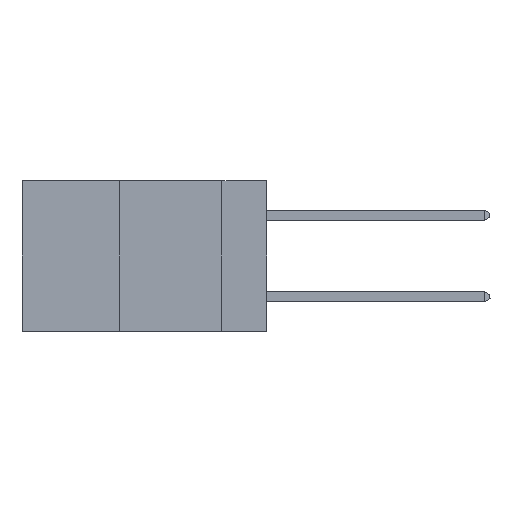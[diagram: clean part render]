
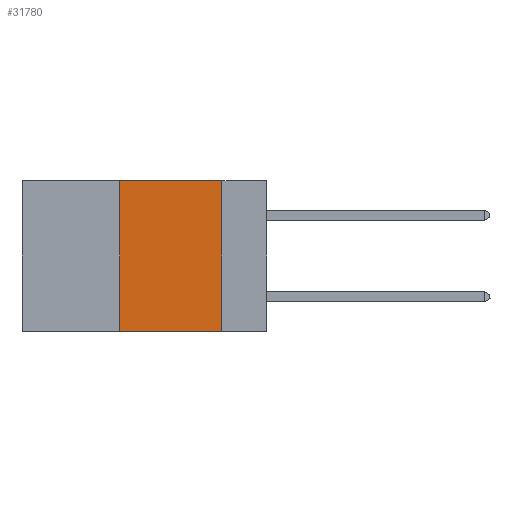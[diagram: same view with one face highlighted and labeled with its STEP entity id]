
A CAD part, left-side view. The second image highlights one B-rep face of the part: STEP entity #31780.
In plain terms, the highlighted planar face has unit normal (-1, 0, 0).
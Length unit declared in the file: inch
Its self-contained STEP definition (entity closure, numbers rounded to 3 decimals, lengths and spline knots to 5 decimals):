
#160 = CARTESIAN_POINT ( 'NONE',  ( 0., 0.6, 0. ) ) ;
#2455 = DIRECTION ( 'NONE',  ( 0., -1., 0. ) ) ;
#2839 = LINE ( 'NONE', #28168, #29266 ) ;
#3097 = ORIENTED_EDGE ( 'NONE', *, *, #26036, .F. ) ;
#4173 = FACE_OUTER_BOUND ( 'NONE', #17280, .T. ) ;
#4982 = VERTEX_POINT ( 'NONE', #21411 ) ;
#5600 = DIRECTION ( 'NONE',  ( 0., 0., -1. ) ) ;
#5843 = ORIENTED_EDGE ( 'NONE', *, *, #27951, .F. ) ;
#10072 = DIRECTION ( 'NONE',  ( 0., -1., 0. ) ) ;
#10886 = VECTOR ( 'NONE', #22219, 39.37008 ) ;
#11198 = DIRECTION ( 'NONE',  ( 1., 0., 0. ) ) ;
#13340 = LINE ( 'NONE', #160, #28936 ) ;
#13749 = DIRECTION ( 'NONE',  ( 0., 0., -1. ) ) ;
#14373 = ORIENTED_EDGE ( 'NONE', *, *, #21920, .T. ) ;
#15315 = ORIENTED_EDGE ( 'NONE', *, *, #31547, .F. ) ;
#15418 = CARTESIAN_POINT ( 'NONE',  ( 0., 0.11, 0. ) ) ;
#17280 = EDGE_LOOP ( 'NONE', ( #15315, #3097, #5843, #14373 ) ) ;
#18230 = VERTEX_POINT ( 'NONE', #19538 ) ;
#19538 = CARTESIAN_POINT ( 'NONE',  ( 0., 0.11, 0. ) ) ;
#21346 = PLANE ( 'NONE',  #22040 ) ;
#21411 = CARTESIAN_POINT ( 'NONE',  ( 0., 0.36, 0. ) ) ;
#21793 = VERTEX_POINT ( 'NONE', #27636 ) ;
#21920 = EDGE_CURVE ( 'NONE', #22216, #21793, #2839, .T. ) ;
#22040 = AXIS2_PLACEMENT_3D ( 'NONE', #23917, #11198, #13749 ) ;
#22216 = VERTEX_POINT ( 'NONE', #29173 ) ;
#22219 = DIRECTION ( 'NONE',  ( 0., 0., 1. ) ) ;
#22330 = CARTESIAN_POINT ( 'NONE',  ( 0., 0.36, 0. ) ) ;
#22848 = LINE ( 'NONE', #22330, #10886 ) ;
#23358 = VECTOR ( 'NONE', #5600, 39.37008 ) ;
#23803 = LINE ( 'NONE', #15418, #23358 ) ;
#23917 = CARTESIAN_POINT ( 'NONE',  ( 0., 0.6, 0. ) ) ;
#26036 = EDGE_CURVE ( 'NONE', #4982, #18230, #13340, .T. ) ;
#27636 = CARTESIAN_POINT ( 'NONE',  ( 0., 0.11, -0.37 ) ) ;
#27951 = EDGE_CURVE ( 'NONE', #22216, #4982, #22848, .T. ) ;
#28168 = CARTESIAN_POINT ( 'NONE',  ( 0., 0.6, -0.37 ) ) ;
#28936 = VECTOR ( 'NONE', #10072, 39.37008 ) ;
#29173 = CARTESIAN_POINT ( 'NONE',  ( 0., 0.36, -0.37 ) ) ;
#29266 = VECTOR ( 'NONE', #2455, 39.37008 ) ;
#31547 = EDGE_CURVE ( 'NONE', #18230, #21793, #23803, .T. ) ;
#31780 = ADVANCED_FACE ( 'NONE', ( #4173 ), #21346, .F. ) ;
